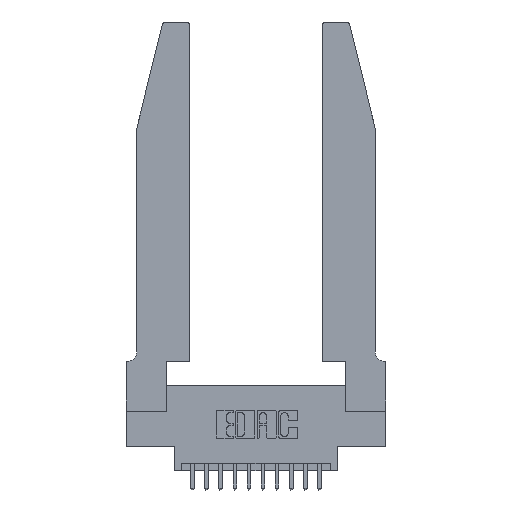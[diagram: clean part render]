
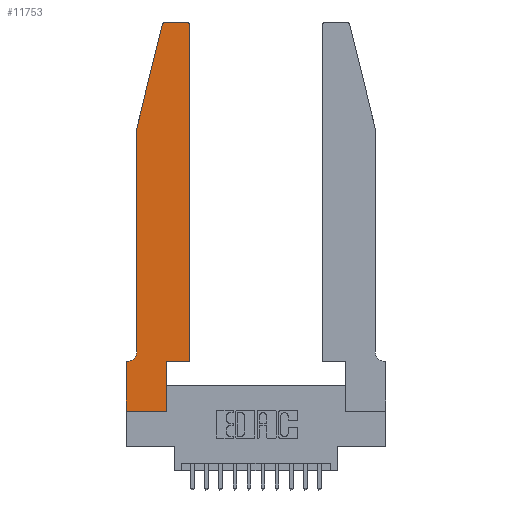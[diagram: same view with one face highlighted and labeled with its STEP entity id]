
A CAD part, top view. The second image highlights one B-rep face of the part: STEP entity #11753.
In plain terms, the highlighted planar face has unit normal (0, 0, 1).
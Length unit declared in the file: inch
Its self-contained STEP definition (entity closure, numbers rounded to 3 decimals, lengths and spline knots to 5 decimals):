
#308 = CARTESIAN_POINT ( 'NONE',  ( 0.284, 2.75, 0.37 ) ) ;
#380 = CARTESIAN_POINT ( 'NONE',  ( 0.2605, 2.75, 0.37 ) ) ;
#424 = EDGE_CURVE ( 'NONE', #5418, #2712, #16541, .T. ) ;
#523 = VERTEX_POINT ( 'NONE', #14859 ) ;
#805 = VERTEX_POINT ( 'NONE', #819 ) ;
#819 = CARTESIAN_POINT ( 'NONE',  ( 0.4505, 2.72, 0.37 ) ) ;
#1378 = ORIENTED_EDGE ( 'NONE', *, *, #8043, .T. ) ;
#1533 = EDGE_CURVE ( 'NONE', #2712, #523, #5865, .T. ) ;
#1816 = EDGE_LOOP ( 'NONE', ( #11060, #7399, #1378, #3282, #1898, #9823, #15288, #14988, #12251, #11359, #14014, #9720 ) ) ;
#1838 = CARTESIAN_POINT ( 'NONE',  ( 0.284, 2.72, 0.37 ) ) ;
#1898 = ORIENTED_EDGE ( 'NONE', *, *, #14186, .T. ) ;
#1946 = CARTESIAN_POINT ( 'NONE',  ( 0.4505, 0.35, 0.37 ) ) ;
#2365 = CIRCLE ( 'NONE', #9443, 0.03 ) ;
#2701 = VECTOR ( 'NONE', #10601, 39.37008 ) ;
#2712 = VERTEX_POINT ( 'NONE', #6296 ) ;
#2870 = VECTOR ( 'NONE', #4382, 39.37008 ) ;
#2893 = CARTESIAN_POINT ( 'NONE',  ( 0.0755, 2., 0.37 ) ) ;
#3001 = CARTESIAN_POINT ( 'NONE',  ( 0.2865, 0., 0.37 ) ) ;
#3062 = LINE ( 'NONE', #1946, #9724 ) ;
#3123 = EDGE_CURVE ( 'NONE', #523, #4040, #3689, .T. ) ;
#3240 = DIRECTION ( 'NONE',  ( 1., 0., 0. ) ) ;
#3282 = ORIENTED_EDGE ( 'NONE', *, *, #5129, .T. ) ;
#3330 = DIRECTION ( 'NONE',  ( 0., 1., 0. ) ) ;
#3518 = CARTESIAN_POINT ( 'NONE',  ( 0.25487, 2.72718, 0.37 ) ) ;
#3689 = LINE ( 'NONE', #6242, #17042 ) ;
#4040 = VERTEX_POINT ( 'NONE', #3001 ) ;
#4108 = AXIS2_PLACEMENT_3D ( 'NONE', #14841, #7210, #16125 ) ;
#4112 = LINE ( 'NONE', #7521, #10699 ) ;
#4382 = DIRECTION ( 'NONE',  ( 0., -1., 0. ) ) ;
#4710 = EDGE_CURVE ( 'NONE', #13225, #14739, #12652, .T. ) ;
#5129 = EDGE_CURVE ( 'NONE', #15772, #12396, #6510, .T. ) ;
#5263 = CARTESIAN_POINT ( 'NONE',  ( 0.4505, 0.35, 0.37 ) ) ;
#5418 = VERTEX_POINT ( 'NONE', #7645 ) ;
#5654 = EDGE_CURVE ( 'NONE', #9716, #15194, #6493, .T. ) ;
#5787 = VECTOR ( 'NONE', #8546, 39.37008 ) ;
#5865 = LINE ( 'NONE', #7104, #12317 ) ;
#6002 = DIRECTION ( 'NONE',  ( 1., 0., 0. ) ) ;
#6005 = CIRCLE ( 'NONE', #4108, 0.03 ) ;
#6090 = EDGE_CURVE ( 'NONE', #4040, #9716, #4112, .T. ) ;
#6163 = DIRECTION ( 'NONE',  ( 0., 1., 0. ) ) ;
#6242 = CARTESIAN_POINT ( 'NONE',  ( 0., 0., 0.37 ) ) ;
#6296 = CARTESIAN_POINT ( 'NONE',  ( 0., 0.35, 0.37 ) ) ;
#6493 = LINE ( 'NONE', #5263, #16288 ) ;
#6510 = LINE ( 'NONE', #16047, #2870 ) ;
#6791 = CARTESIAN_POINT ( 'NONE',  ( 0.2865, 0.35, 0.37 ) ) ;
#6970 = CIRCLE ( 'NONE', #14367, 0.07 ) ;
#7104 = CARTESIAN_POINT ( 'NONE',  ( 0., 0., 0.37 ) ) ;
#7122 = DIRECTION ( 'NONE',  ( 0., -1., 0. ) ) ;
#7183 = AXIS2_PLACEMENT_3D ( 'NONE', #11099, #7309, #16221 ) ;
#7210 = DIRECTION ( 'NONE',  ( 0., 0., 1. ) ) ;
#7309 = DIRECTION ( 'NONE',  ( 0., 0., 1. ) ) ;
#7399 = ORIENTED_EDGE ( 'NONE', *, *, #12234, .T. ) ;
#7516 = CARTESIAN_POINT ( 'NONE',  ( 0.0055, 0.42, 0.37 ) ) ;
#7521 = CARTESIAN_POINT ( 'NONE',  ( 0.2865, 0.35, 0.37 ) ) ;
#7645 = CARTESIAN_POINT ( 'NONE',  ( 0.0055, 0.35, 0.37 ) ) ;
#7762 = VERTEX_POINT ( 'NONE', #3518 ) ;
#8043 = EDGE_CURVE ( 'NONE', #7762, #15772, #8282, .T. ) ;
#8282 = LINE ( 'NONE', #2893, #11671 ) ;
#8546 = DIRECTION ( 'NONE',  ( -1., 0., 0. ) ) ;
#8777 = DIRECTION ( 'NONE',  ( -1., 0., 0. ) ) ;
#9443 = AXIS2_PLACEMENT_3D ( 'NONE', #1838, #11121, #3240 ) ;
#9716 = VERTEX_POINT ( 'NONE', #6791 ) ;
#9720 = ORIENTED_EDGE ( 'NONE', *, *, #12189, .T. ) ;
#9724 = VECTOR ( 'NONE', #3330, 39.37008 ) ;
#9823 = ORIENTED_EDGE ( 'NONE', *, *, #424, .T. ) ;
#10601 = DIRECTION ( 'NONE',  ( -1., 0., 0. ) ) ;
#10699 = VECTOR ( 'NONE', #6163, 39.37008 ) ;
#10804 = DIRECTION ( 'NONE',  ( -0.239, -0.971, 0. ) ) ;
#10881 = CARTESIAN_POINT ( 'NONE',  ( 0.0755, 0.35, 0.37 ) ) ;
#11060 = ORIENTED_EDGE ( 'NONE', *, *, #4710, .T. ) ;
#11099 = CARTESIAN_POINT ( 'NONE',  ( 0., 0.35, 0.37 ) ) ;
#11121 = DIRECTION ( 'NONE',  ( 0., 0., 1. ) ) ;
#11143 = FACE_OUTER_BOUND ( 'NONE', #1816, .T. ) ;
#11336 = CARTESIAN_POINT ( 'NONE',  ( 0.4505, 0.35, 0.37 ) ) ;
#11359 = ORIENTED_EDGE ( 'NONE', *, *, #5654, .T. ) ;
#11671 = VECTOR ( 'NONE', #10804, 39.37008 ) ;
#11753 = ADVANCED_FACE ( 'NONE', ( #11143 ), #14926, .T. ) ;
#12189 = EDGE_CURVE ( 'NONE', #805, #13225, #6005, .T. ) ;
#12234 = EDGE_CURVE ( 'NONE', #14739, #7762, #2365, .T. ) ;
#12251 = ORIENTED_EDGE ( 'NONE', *, *, #6090, .T. ) ;
#12317 = VECTOR ( 'NONE', #7122, 39.37008 ) ;
#12396 = VERTEX_POINT ( 'NONE', #16509 ) ;
#12652 = LINE ( 'NONE', #380, #5787 ) ;
#13141 = DIRECTION ( 'NONE',  ( 1., 0., 0. ) ) ;
#13225 = VERTEX_POINT ( 'NONE', #16817 ) ;
#14014 = ORIENTED_EDGE ( 'NONE', *, *, #17066, .T. ) ;
#14186 = EDGE_CURVE ( 'NONE', #12396, #5418, #6970, .T. ) ;
#14367 = AXIS2_PLACEMENT_3D ( 'NONE', #7516, #16404, #8777 ) ;
#14739 = VERTEX_POINT ( 'NONE', #308 ) ;
#14841 = CARTESIAN_POINT ( 'NONE',  ( 0.4205, 2.72, 0.37 ) ) ;
#14859 = CARTESIAN_POINT ( 'NONE',  ( 0., 0., 0.37 ) ) ;
#14926 = PLANE ( 'NONE',  #7183 ) ;
#14988 = ORIENTED_EDGE ( 'NONE', *, *, #3123, .T. ) ;
#15194 = VERTEX_POINT ( 'NONE', #11336 ) ;
#15288 = ORIENTED_EDGE ( 'NONE', *, *, #1533, .T. ) ;
#15772 = VERTEX_POINT ( 'NONE', #16865 ) ;
#16047 = CARTESIAN_POINT ( 'NONE',  ( 0.0755, 2., 0.37 ) ) ;
#16125 = DIRECTION ( 'NONE',  ( 1., 0., 0. ) ) ;
#16221 = DIRECTION ( 'NONE',  ( 1., 0., 0. ) ) ;
#16288 = VECTOR ( 'NONE', #13141, 39.37008 ) ;
#16404 = DIRECTION ( 'NONE',  ( 0., 0., -1. ) ) ;
#16509 = CARTESIAN_POINT ( 'NONE',  ( 0.0755, 0.42, 0.37 ) ) ;
#16541 = LINE ( 'NONE', #10881, #2701 ) ;
#16817 = CARTESIAN_POINT ( 'NONE',  ( 0.4205, 2.75, 0.37 ) ) ;
#16865 = CARTESIAN_POINT ( 'NONE',  ( 0.0755, 2., 0.37 ) ) ;
#17042 = VECTOR ( 'NONE', #6002, 39.37008 ) ;
#17066 = EDGE_CURVE ( 'NONE', #15194, #805, #3062, .T. ) ;
